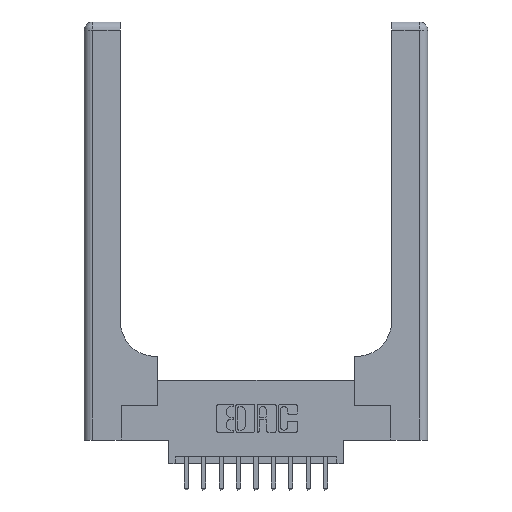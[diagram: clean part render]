
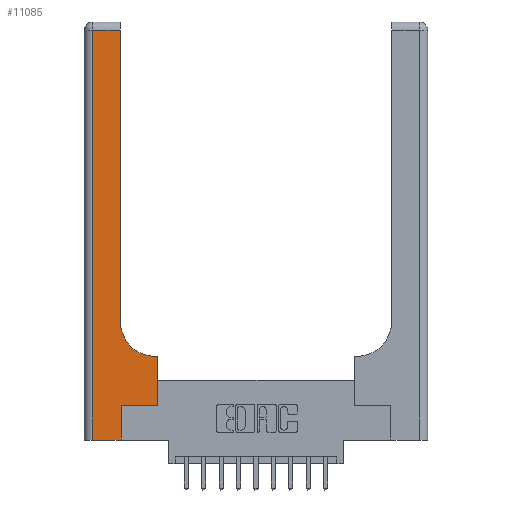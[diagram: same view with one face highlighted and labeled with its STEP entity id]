
A CAD part, top view. The second image highlights one B-rep face of the part: STEP entity #11085.
In plain terms, the highlighted planar face has unit normal (0, 0, 1).
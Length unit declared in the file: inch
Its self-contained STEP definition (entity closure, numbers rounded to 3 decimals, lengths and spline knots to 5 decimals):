
#549 = LINE ( 'NONE', #3332, #6759 ) ;
#577 = CARTESIAN_POINT ( 'NONE',  ( 0.528, 0.25, 0.37 ) ) ;
#726 = CIRCLE ( 'NONE', #8494, 0.25 ) ;
#834 = EDGE_CURVE ( 'NONE', #5805, #2649, #3664, .T. ) ;
#862 = LINE ( 'NONE', #2656, #9914 ) ;
#1049 = CARTESIAN_POINT ( 'NONE',  ( 0.265, 0.25, 0.37 ) ) ;
#1338 = DIRECTION ( 'NONE',  ( 0., 0., -1. ) ) ;
#1384 = CARTESIAN_POINT ( 'NONE',  ( 0.528, 0.25, 0.37 ) ) ;
#1438 = DIRECTION ( 'NONE',  ( -1., 0., 0. ) ) ;
#1545 = EDGE_CURVE ( 'NONE', #12271, #13901, #549, .T. ) ;
#1968 = DIRECTION ( 'NONE',  ( 0., 1., 0. ) ) ;
#2027 = FACE_OUTER_BOUND ( 'NONE', #13591, .T. ) ;
#2210 = AXIS2_PLACEMENT_3D ( 'NONE', #5681, #15309, #8156 ) ;
#2531 = CARTESIAN_POINT ( 'NONE',  ( 0.26, 0.6, 0.37 ) ) ;
#2576 = CARTESIAN_POINT ( 'NONE',  ( 0.06, 0., 0.37 ) ) ;
#2594 = ORIENTED_EDGE ( 'NONE', *, *, #1545, .T. ) ;
#2649 = VERTEX_POINT ( 'NONE', #2576 ) ;
#2656 = CARTESIAN_POINT ( 'NONE',  ( 0., 0., 0.37 ) ) ;
#2730 = CARTESIAN_POINT ( 'NONE',  ( 0.26, 3., 0.37 ) ) ;
#3274 = CARTESIAN_POINT ( 'NONE',  ( 0.26, 2.94, 0.37 ) ) ;
#3332 = CARTESIAN_POINT ( 'NONE',  ( 0.265, 0., 0.37 ) ) ;
#3490 = CARTESIAN_POINT ( 'NONE',  ( 0.51, 0.6, 0.37 ) ) ;
#3664 = LINE ( 'NONE', #10384, #9821 ) ;
#3827 = CARTESIAN_POINT ( 'NONE',  ( 0.265, 0., 0.37 ) ) ;
#3887 = CARTESIAN_POINT ( 'NONE',  ( 0., 2.94, 0.37 ) ) ;
#4626 = VECTOR ( 'NONE', #9985, 39.37008 ) ;
#4683 = ORIENTED_EDGE ( 'NONE', *, *, #9704, .T. ) ;
#4883 = DIRECTION ( 'NONE',  ( 1., 0., 0. ) ) ;
#4932 = VERTEX_POINT ( 'NONE', #577 ) ;
#5681 = CARTESIAN_POINT ( 'NONE',  ( 0., 3., 0.37 ) ) ;
#5805 = VERTEX_POINT ( 'NONE', #10670 ) ;
#5893 = DIRECTION ( 'NONE',  ( -1., 0., 0. ) ) ;
#6128 = LINE ( 'NONE', #3887, #14967 ) ;
#6299 = VERTEX_POINT ( 'NONE', #12514 ) ;
#6759 = VECTOR ( 'NONE', #1968, 39.37008 ) ;
#6993 = VECTOR ( 'NONE', #5893, 39.37008 ) ;
#7218 = ORIENTED_EDGE ( 'NONE', *, *, #15206, .T. ) ;
#7382 = LINE ( 'NONE', #2531, #6993 ) ;
#7934 = LINE ( 'NONE', #1384, #4626 ) ;
#8082 = DIRECTION ( 'NONE',  ( 0., -1., 0. ) ) ;
#8156 = DIRECTION ( 'NONE',  ( -1., 0., 0. ) ) ;
#8484 = LINE ( 'NONE', #10924, #11253 ) ;
#8494 = AXIS2_PLACEMENT_3D ( 'NONE', #8758, #1338, #9945 ) ;
#8758 = CARTESIAN_POINT ( 'NONE',  ( 0.51, 0.85, 0.37 ) ) ;
#8902 = DIRECTION ( 'NONE',  ( 0., 1., 0. ) ) ;
#9269 = ORIENTED_EDGE ( 'NONE', *, *, #834, .T. ) ;
#9321 = CARTESIAN_POINT ( 'NONE',  ( 0.26, 0.85, 0.37 ) ) ;
#9469 = VERTEX_POINT ( 'NONE', #3274 ) ;
#9604 = VECTOR ( 'NONE', #8902, 39.37008 ) ;
#9704 = EDGE_CURVE ( 'NONE', #4932, #6299, #7934, .T. ) ;
#9778 = EDGE_CURVE ( 'NONE', #12643, #9469, #9972, .T. ) ;
#9821 = VECTOR ( 'NONE', #8082, 39.37008 ) ;
#9914 = VECTOR ( 'NONE', #12421, 39.37008 ) ;
#9945 = DIRECTION ( 'NONE',  ( 1., 0., 0. ) ) ;
#9972 = LINE ( 'NONE', #2730, #9604 ) ;
#9985 = DIRECTION ( 'NONE',  ( 0., 1., 0. ) ) ;
#10384 = CARTESIAN_POINT ( 'NONE',  ( 0.06, 3., 0.37 ) ) ;
#10647 = ORIENTED_EDGE ( 'NONE', *, *, #11727, .T. ) ;
#10670 = CARTESIAN_POINT ( 'NONE',  ( 0.06, 2.94, 0.37 ) ) ;
#10924 = CARTESIAN_POINT ( 'NONE',  ( 0.265, 0.25, 0.37 ) ) ;
#11085 = ADVANCED_FACE ( 'NONE', ( #2027 ), #14114, .F. ) ;
#11253 = VECTOR ( 'NONE', #4883, 39.37008 ) ;
#11727 = EDGE_CURVE ( 'NONE', #2649, #12271, #862, .T. ) ;
#12271 = VERTEX_POINT ( 'NONE', #3827 ) ;
#12314 = EDGE_CURVE ( 'NONE', #9469, #5805, #6128, .T. ) ;
#12421 = DIRECTION ( 'NONE',  ( 1., 0., 0. ) ) ;
#12514 = CARTESIAN_POINT ( 'NONE',  ( 0.528, 0.6, 0.37 ) ) ;
#12643 = VERTEX_POINT ( 'NONE', #9321 ) ;
#13591 = EDGE_LOOP ( 'NONE', ( #13933, #14276, #9269, #10647, #2594, #7218, #4683, #14443, #14757 ) ) ;
#13818 = EDGE_CURVE ( 'NONE', #6299, #13897, #7382, .T. ) ;
#13897 = VERTEX_POINT ( 'NONE', #3490 ) ;
#13901 = VERTEX_POINT ( 'NONE', #1049 ) ;
#13933 = ORIENTED_EDGE ( 'NONE', *, *, #9778, .T. ) ;
#14114 = PLANE ( 'NONE',  #2210 ) ;
#14276 = ORIENTED_EDGE ( 'NONE', *, *, #12314, .T. ) ;
#14443 = ORIENTED_EDGE ( 'NONE', *, *, #13818, .T. ) ;
#14757 = ORIENTED_EDGE ( 'NONE', *, *, #15311, .T. ) ;
#14967 = VECTOR ( 'NONE', #1438, 39.37008 ) ;
#15206 = EDGE_CURVE ( 'NONE', #13901, #4932, #8484, .T. ) ;
#15309 = DIRECTION ( 'NONE',  ( 0., 0., -1. ) ) ;
#15311 = EDGE_CURVE ( 'NONE', #13897, #12643, #726, .T. ) ;
